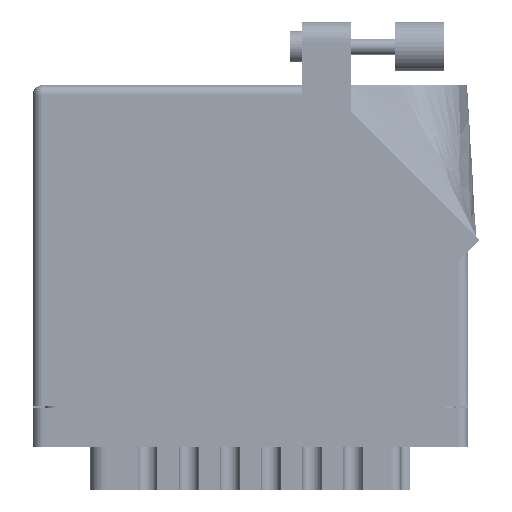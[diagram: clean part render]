
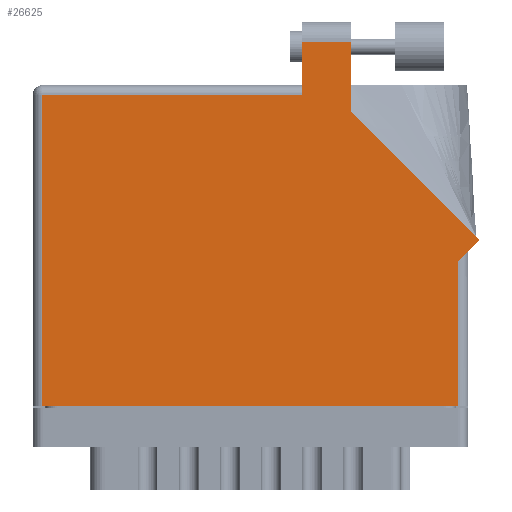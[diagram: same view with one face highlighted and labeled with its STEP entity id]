
A CAD part, front view. The second image highlights one B-rep face of the part: STEP entity #26625.
In plain terms, the highlighted face is planar.
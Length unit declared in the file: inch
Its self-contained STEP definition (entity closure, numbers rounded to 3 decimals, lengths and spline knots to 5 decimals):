
#2750 = LINE ( 'NONE', #73067, #38815 ) ;
#5631 = VECTOR ( 'NONE', #86847, 39.37008 ) ;
#7529 = ORIENTED_EDGE ( 'NONE', *, *, #66100, .T. ) ;
#8441 = EDGE_CURVE ( 'NONE', #43100, #63454, #93024, .T. ) ;
#10329 = ORIENTED_EDGE ( 'NONE', *, *, #27471, .T. ) ;
#10361 = ORIENTED_EDGE ( 'NONE', *, *, #59870, .T. ) ;
#11379 = DIRECTION ( 'NONE',  ( -1., 0., 0. ) ) ;
#11563 = EDGE_CURVE ( 'NONE', #48789, #47698, #14368, .T. ) ;
#12038 = CARTESIAN_POINT ( 'NONE',  ( 0.062, 1.968, 0. ) ) ;
#12587 = DIRECTION ( 'NONE',  ( -0.707, 0.707, 0. ) ) ;
#13867 = CARTESIAN_POINT ( 'NONE',  ( 2.82571, 1.05071, 0. ) ) ;
#14368 = LINE ( 'NONE', #46132, #93705 ) ;
#15028 = VERTEX_POINT ( 'NONE', #86211 ) ;
#16037 = LINE ( 'NONE', #13867, #77832 ) ;
#20715 = CARTESIAN_POINT ( 'NONE',  ( 2.693, 0.98, 0. ) ) ;
#21011 = CARTESIAN_POINT ( 'NONE',  ( 2.693, 0., 0. ) ) ;
#21387 = VECTOR ( 'NONE', #28213, 39.37008 ) ;
#22250 = VERTEX_POINT ( 'NONE', #60610 ) ;
#26625 = ADVANCED_FACE ( 'NONE', ( #94055 ), #26666, .F. ) ;
#26666 = PLANE ( 'NONE',  #35930 ) ;
#26986 = VERTEX_POINT ( 'NONE', #59343 ) ;
#27471 = EDGE_CURVE ( 'NONE', #74376, #43100, #29652, .T. ) ;
#28213 = DIRECTION ( 'NONE',  ( 0., 1., 0. ) ) ;
#29652 = LINE ( 'NONE', #32413, #41328 ) ;
#32413 = CARTESIAN_POINT ( 'NONE',  ( 0.062, 0., 0. ) ) ;
#33039 = CARTESIAN_POINT ( 'NONE',  ( 0.062, 0., 0. ) ) ;
#35009 = EDGE_CURVE ( 'NONE', #63454, #48789, #55242, .T. ) ;
#35930 = AXIS2_PLACEMENT_3D ( 'NONE', #78398, #70285, #11379 ) ;
#37123 = CARTESIAN_POINT ( 'NONE',  ( 1.705, 2.03, 0. ) ) ;
#38627 = ORIENTED_EDGE ( 'NONE', *, *, #75136, .T. ) ;
#38815 = VECTOR ( 'NONE', #48823, 39.37008 ) ;
#38973 = DIRECTION ( 'NONE',  ( 0.707, 0.707, 0. ) ) ;
#40559 = DIRECTION ( 'NONE',  ( 0., -1., 0. ) ) ;
#41012 = ORIENTED_EDGE ( 'NONE', *, *, #78704, .T. ) ;
#41328 = VECTOR ( 'NONE', #40559, 39.37008 ) ;
#42203 = CARTESIAN_POINT ( 'NONE',  ( 2.012, 1.86442, 0. ) ) ;
#43100 = VERTEX_POINT ( 'NONE', #33039 ) ;
#43245 = CARTESIAN_POINT ( 'NONE',  ( 2.012, 1.86442, 0. ) ) ;
#45365 = DIRECTION ( 'NONE',  ( 1., 0., 0. ) ) ;
#46132 = CARTESIAN_POINT ( 'NONE',  ( 2.755, 0.98, 0. ) ) ;
#47698 = VERTEX_POINT ( 'NONE', #67700 ) ;
#48255 = VECTOR ( 'NONE', #61246, 39.37008 ) ;
#48789 = VERTEX_POINT ( 'NONE', #58393 ) ;
#48823 = DIRECTION ( 'NONE',  ( -1., 0., 0. ) ) ;
#49005 = EDGE_CURVE ( 'NONE', #26986, #74376, #82724, .T. ) ;
#55242 = LINE ( 'NONE', #20715, #21387 ) ;
#57959 = LINE ( 'NONE', #42203, #5631 ) ;
#58393 = CARTESIAN_POINT ( 'NONE',  ( 2.693, 0.918, 0. ) ) ;
#59343 = CARTESIAN_POINT ( 'NONE',  ( 1.705, 1.968, 0. ) ) ;
#59870 = EDGE_CURVE ( 'NONE', #82385, #22250, #57959, .T. ) ;
#60610 = CARTESIAN_POINT ( 'NONE',  ( 2.012, 2.305, 0. ) ) ;
#61246 = DIRECTION ( 'NONE',  ( 0., -1., 0. ) ) ;
#61948 = ORIENTED_EDGE ( 'NONE', *, *, #35009, .T. ) ;
#63454 = VERTEX_POINT ( 'NONE', #21011 ) ;
#64096 = VECTOR ( 'NONE', #90349, 39.37008 ) ;
#64927 = ORIENTED_EDGE ( 'NONE', *, *, #8441, .T. ) ;
#65301 = CARTESIAN_POINT ( 'NONE',  ( 0., 0., 0. ) ) ;
#66100 = EDGE_CURVE ( 'NONE', #15028, #26986, #66940, .T. ) ;
#66940 = LINE ( 'NONE', #37123, #48255 ) ;
#67700 = CARTESIAN_POINT ( 'NONE',  ( 2.82571, 1.05071, 0. ) ) ;
#67777 = CARTESIAN_POINT ( 'NONE',  ( 0., 1.968, 0. ) ) ;
#70285 = DIRECTION ( 'NONE',  ( 0., 0., -1. ) ) ;
#73067 = CARTESIAN_POINT ( 'NONE',  ( 1.705, 2.305, 0. ) ) ;
#74376 = VERTEX_POINT ( 'NONE', #12038 ) ;
#75136 = EDGE_CURVE ( 'NONE', #22250, #15028, #2750, .T. ) ;
#76570 = VECTOR ( 'NONE', #45365, 39.37008 ) ;
#77832 = VECTOR ( 'NONE', #12587, 39.37008 ) ;
#78398 = CARTESIAN_POINT ( 'NONE',  ( 0., 2.03, 0. ) ) ;
#78704 = EDGE_CURVE ( 'NONE', #47698, #82385, #16037, .T. ) ;
#82385 = VERTEX_POINT ( 'NONE', #43245 ) ;
#82724 = LINE ( 'NONE', #67777, #64096 ) ;
#85669 = ORIENTED_EDGE ( 'NONE', *, *, #11563, .T. ) ;
#86211 = CARTESIAN_POINT ( 'NONE',  ( 1.705, 2.305, 0. ) ) ;
#86847 = DIRECTION ( 'NONE',  ( 0., 1., 0. ) ) ;
#87828 = ORIENTED_EDGE ( 'NONE', *, *, #49005, .T. ) ;
#90349 = DIRECTION ( 'NONE',  ( -1., 0., 0. ) ) ;
#93024 = LINE ( 'NONE', #65301, #76570 ) ;
#93705 = VECTOR ( 'NONE', #38973, 39.37008 ) ;
#94055 = FACE_OUTER_BOUND ( 'NONE', #96470, .T. ) ;
#96470 = EDGE_LOOP ( 'NONE', ( #10361, #38627, #7529, #87828, #10329, #64927, #61948, #85669, #41012 ) ) ;
